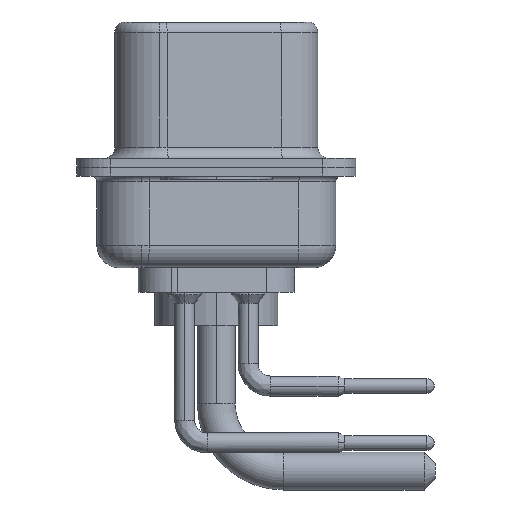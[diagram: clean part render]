
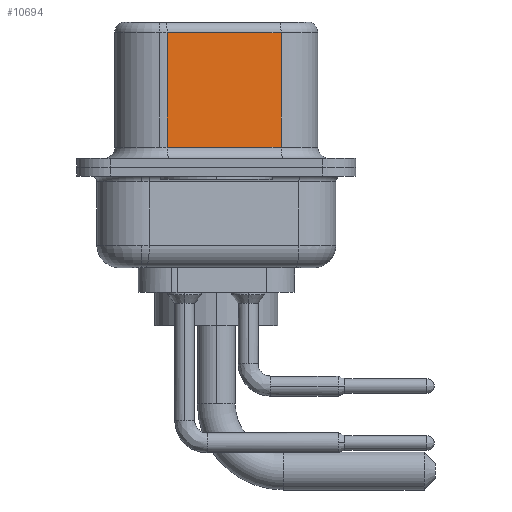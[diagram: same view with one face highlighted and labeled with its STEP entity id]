
A CAD part, left-side view. The second image highlights one B-rep face of the part: STEP entity #10694.
In plain terms, the highlighted planar face has unit normal (-0.985, -0.174, 0).
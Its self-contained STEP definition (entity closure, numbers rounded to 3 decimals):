
#61 = DIRECTION ( 'NONE',  ( 0., 0., -1. ) ) ;
#325 = EDGE_CURVE ( 'NONE', #11883, #2779, #11082, .T. ) ;
#353 = EDGE_LOOP ( 'NONE', ( #8897, #16592, #4258, #9232 ) ) ;
#1245 = VERTEX_POINT ( 'NONE', #5167 ) ;
#1324 = LINE ( 'NONE', #7974, #8178 ) ;
#2734 = LINE ( 'NONE', #17280, #7137 ) ;
#2779 = VERTEX_POINT ( 'NONE', #3169 ) ;
#3169 = CARTESIAN_POINT ( 'NONE',  ( 4.58, -2.897, 0.9 ) ) ;
#3410 = LINE ( 'NONE', #11741, #16714 ) ;
#4258 = ORIENTED_EDGE ( 'NONE', *, *, #15647, .T. ) ;
#5032 = VECTOR ( 'NONE', #11915, 1000. ) ;
#5167 = CARTESIAN_POINT ( 'NONE',  ( 4.58, -2.897, 6.02 ) ) ;
#6858 = CARTESIAN_POINT ( 'NONE',  ( 3.68, 2.203, 6.02 ) ) ;
#7137 = VECTOR ( 'NONE', #61, 1000. ) ;
#7974 = CARTESIAN_POINT ( 'NONE',  ( 4.58, -2.897, 6.02 ) ) ;
#8178 = VECTOR ( 'NONE', #17462, 1000. ) ;
#8897 = ORIENTED_EDGE ( 'NONE', *, *, #14551, .F. ) ;
#9012 = CARTESIAN_POINT ( 'NONE',  ( 4.58, -2.897, 6.52 ) ) ;
#9232 = ORIENTED_EDGE ( 'NONE', *, *, #325, .T. ) ;
#10632 = AXIS2_PLACEMENT_3D ( 'NONE', #9012, #17081, #15748 ) ;
#10694 = ADVANCED_FACE ( 'NONE', ( #11680 ), #14067, .F. ) ;
#11082 = LINE ( 'NONE', #12088, #5032 ) ;
#11680 = FACE_OUTER_BOUND ( 'NONE', #353, .T. ) ;
#11741 = CARTESIAN_POINT ( 'NONE',  ( 4.58, -2.897, 6.52 ) ) ;
#11883 = VERTEX_POINT ( 'NONE', #12845 ) ;
#11915 = DIRECTION ( 'NONE',  ( 0.174, -0.985, 0. ) ) ;
#12088 = CARTESIAN_POINT ( 'NONE',  ( 4.58, -2.897, 0.9 ) ) ;
#12674 = VERTEX_POINT ( 'NONE', #6858 ) ;
#12845 = CARTESIAN_POINT ( 'NONE',  ( 3.68, 2.203, 0.9 ) ) ;
#13452 = EDGE_CURVE ( 'NONE', #1245, #12674, #1324, .T. ) ;
#14067 = PLANE ( 'NONE',  #10632 ) ;
#14551 = EDGE_CURVE ( 'NONE', #1245, #2779, #3410, .T. ) ;
#15647 = EDGE_CURVE ( 'NONE', #12674, #11883, #2734, .T. ) ;
#15748 = DIRECTION ( 'NONE',  ( -0.174, 0.985, 0. ) ) ;
#16592 = ORIENTED_EDGE ( 'NONE', *, *, #13452, .T. ) ;
#16714 = VECTOR ( 'NONE', #17144, 1000. ) ;
#17081 = DIRECTION ( 'NONE',  ( 0.985, 0.174, 0. ) ) ;
#17144 = DIRECTION ( 'NONE',  ( 0., 0., -1. ) ) ;
#17280 = CARTESIAN_POINT ( 'NONE',  ( 3.68, 2.203, 6.52 ) ) ;
#17462 = DIRECTION ( 'NONE',  ( -0.174, 0.985, 0. ) ) ;
